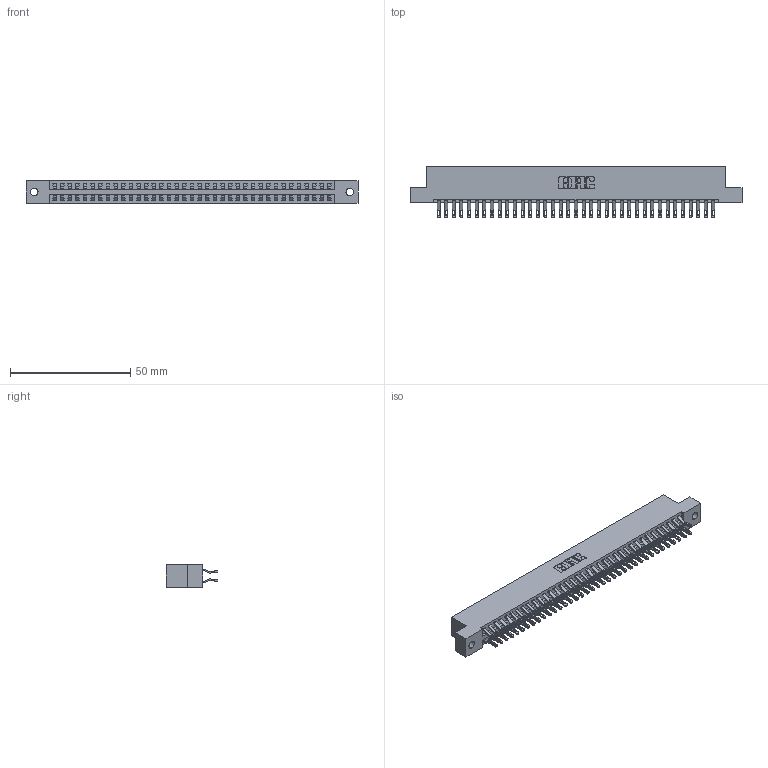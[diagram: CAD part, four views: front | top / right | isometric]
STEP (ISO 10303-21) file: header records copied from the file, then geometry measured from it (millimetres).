
FILE_DESCRIPTION (( 'STEP AP203' ), '1' );
FILE_NAME ('396-074-555-202.STEP', '2018-09-09T12:16:32', ( '' ), ( '' ), 'SwSTEP 2.0', 'SolidWorks 2016', '' );
FILE_SCHEMA (( 'CONFIG_CONTROL_DESIGN' ));
Length unit declared in the file: inch
Products named in the file (3): 396-074-555-202; 345-292-001_555 Tail; 346 Part_Flush Mounting Lugs - 0.128 Dia
Assembly tree (75 placements, depth 2):
  396-074-555-202
    346 Part_Flush Mounting Lugs - 0.128 Dia
    345-292-001_555 Tail  x74
Bounding box: 138.05 x 21.46 x 9.4 mm (x, y, z)
Volume: 13600.6 mm3; surface area: 19112.2 mm2
Topology: 75 solids, 75 shells, 4414 faces, 13871 edges, 9246 vertices
Faces by surface type: plane 2518, cylinder 1896
Entity records: 25149 total; most frequent: CARTESIAN_POINT 4186, ORIENTED_EDGE 4090, DIRECTION 3709, EDGE_CURVE 2045, LINE 1745, VECTOR 1745, VERTEX_POINT 1362, AXIS2_PLACEMENT_3D 982
